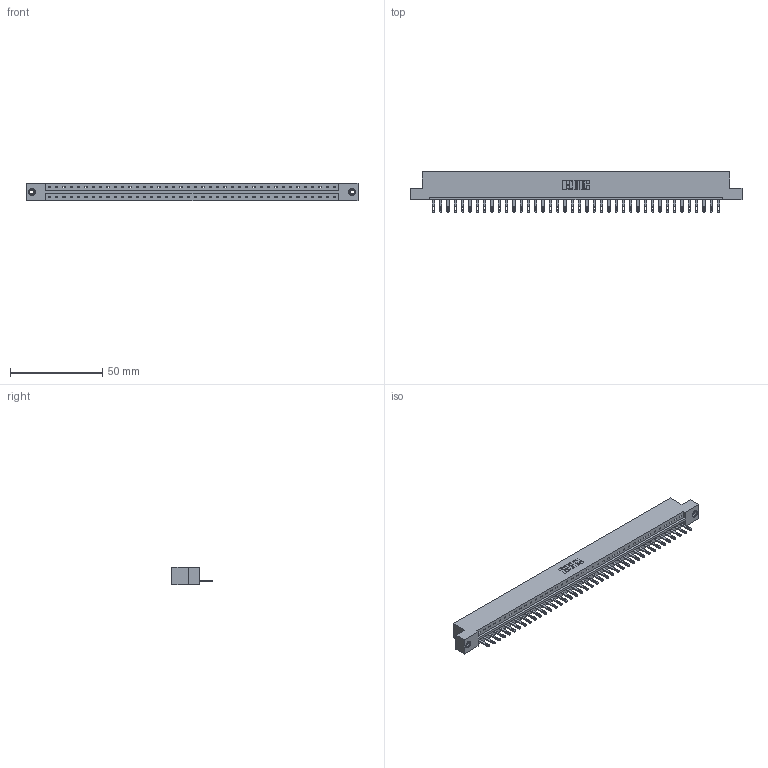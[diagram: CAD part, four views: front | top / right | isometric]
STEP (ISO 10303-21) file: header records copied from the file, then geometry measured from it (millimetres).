
FILE_DESCRIPTION (( 'STEP AP203' ), '1' );
FILE_NAME ('333-040-500-108.STEP', '2018-08-03T13:21:30', ( '' ), ( '' ), 'SwSTEP 2.0', 'SolidWorks 2016', '' );
FILE_SCHEMA (( 'CONFIG_CONTROL_DESIGN' ));
Length unit declared in the file: inch
Products named in the file (4): 333-040-500-108; 333 Part_Flush - .156 Dia - TI; 345-292-001_345-293-100; 345-250-001_345-250-003-102
Assembly tree (43 placements, depth 2):
  333-040-500-108
    333 Part_Flush - .156 Dia - TI
    345-292-001_345-293-100  x40
    345-250-001_345-250-003-102  x2
Bounding box: 180.04 x 21.85 x 9.4 mm (x, y, z)
Volume: 18117.7 mm3; surface area: 19712.9 mm2
Topology: 43 solids, 43 shells, 2334 faces, 7167 edges, 4770 vertices
Faces by surface type: plane 1542, cylinder 776, cone 12, torus 4
Entity records: 25828 total; most frequent: CARTESIAN_POINT 4437, ORIENTED_EDGE 4406, DIRECTION 3781, EDGE_CURVE 2203, LINE 2051, VECTOR 2051, VERTEX_POINT 1464, AXIS2_PLACEMENT_3D 865
